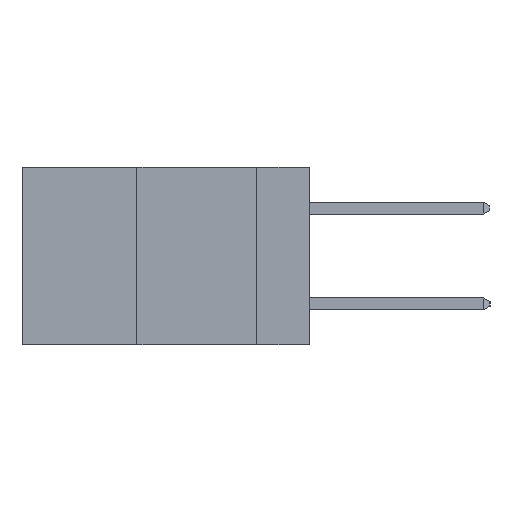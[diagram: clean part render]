
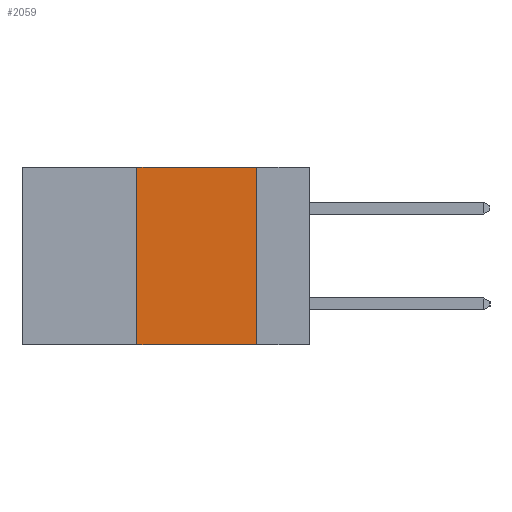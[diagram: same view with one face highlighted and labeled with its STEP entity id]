
A CAD part, left-side view. The second image highlights one B-rep face of the part: STEP entity #2059.
In plain terms, the highlighted planar face has unit normal (-1, 0, 0).
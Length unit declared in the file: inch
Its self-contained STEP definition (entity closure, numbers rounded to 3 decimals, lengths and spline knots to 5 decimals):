
#247 = CARTESIAN_POINT ( 'NONE',  ( 0., 0.36, 0. ) ) ;
#370 = CARTESIAN_POINT ( 'NONE',  ( 0., 0.6, 0. ) ) ;
#443 = LINE ( 'NONE', #370, #8447 ) ;
#1700 = ORIENTED_EDGE ( 'NONE', *, *, #7930, .F. ) ;
#2059 = ADVANCED_FACE ( 'NONE', ( #3210 ), #5375, .F. ) ;
#2315 = DIRECTION ( 'NONE',  ( 0., 0., -1. ) ) ;
#2429 = LINE ( 'NONE', #11252, #8814 ) ;
#2862 = AXIS2_PLACEMENT_3D ( 'NONE', #6428, #8529, #2315 ) ;
#2983 = CARTESIAN_POINT ( 'NONE',  ( 0., 0.36, 0. ) ) ;
#3136 = CARTESIAN_POINT ( 'NONE',  ( 0., 0.11, 0. ) ) ;
#3210 = FACE_OUTER_BOUND ( 'NONE', #4230, .T. ) ;
#3223 = CARTESIAN_POINT ( 'NONE',  ( 0., 0.36, -0.37 ) ) ;
#3445 = CARTESIAN_POINT ( 'NONE',  ( 0., 0.11, -0.37 ) ) ;
#3486 = VERTEX_POINT ( 'NONE', #3445 ) ;
#3592 = VERTEX_POINT ( 'NONE', #2983 ) ;
#3692 = EDGE_CURVE ( 'NONE', #12149, #3486, #2429, .T. ) ;
#3868 = LINE ( 'NONE', #7731, #5164 ) ;
#4230 = EDGE_LOOP ( 'NONE', ( #8853, #12292, #1700, #4834 ) ) ;
#4834 = ORIENTED_EDGE ( 'NONE', *, *, #3692, .T. ) ;
#4853 = EDGE_CURVE ( 'NONE', #9982, #3486, #3868, .T. ) ;
#4954 = LINE ( 'NONE', #247, #9547 ) ;
#5164 = VECTOR ( 'NONE', #6677, 39.37008 ) ;
#5375 = PLANE ( 'NONE',  #2862 ) ;
#6428 = CARTESIAN_POINT ( 'NONE',  ( 0., 0.6, 0. ) ) ;
#6677 = DIRECTION ( 'NONE',  ( 0., 0., -1. ) ) ;
#6832 = DIRECTION ( 'NONE',  ( 0., -1., 0. ) ) ;
#7731 = CARTESIAN_POINT ( 'NONE',  ( 0., 0.11, 0. ) ) ;
#7930 = EDGE_CURVE ( 'NONE', #12149, #3592, #4954, .T. ) ;
#8447 = VECTOR ( 'NONE', #13096, 39.37008 ) ;
#8529 = DIRECTION ( 'NONE',  ( 1., 0., 0. ) ) ;
#8814 = VECTOR ( 'NONE', #6832, 39.37008 ) ;
#8853 = ORIENTED_EDGE ( 'NONE', *, *, #4853, .F. ) ;
#9547 = VECTOR ( 'NONE', #9670, 39.37008 ) ;
#9670 = DIRECTION ( 'NONE',  ( 0., 0., 1. ) ) ;
#9982 = VERTEX_POINT ( 'NONE', #3136 ) ;
#11252 = CARTESIAN_POINT ( 'NONE',  ( 0., 0.6, -0.37 ) ) ;
#11967 = EDGE_CURVE ( 'NONE', #3592, #9982, #443, .T. ) ;
#12149 = VERTEX_POINT ( 'NONE', #3223 ) ;
#12292 = ORIENTED_EDGE ( 'NONE', *, *, #11967, .F. ) ;
#13096 = DIRECTION ( 'NONE',  ( 0., -1., 0. ) ) ;
